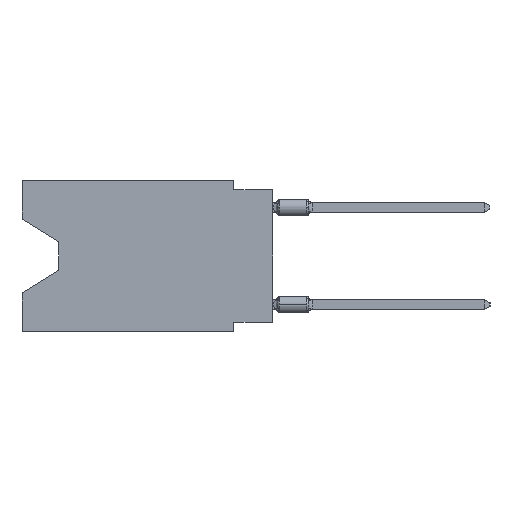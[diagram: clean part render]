
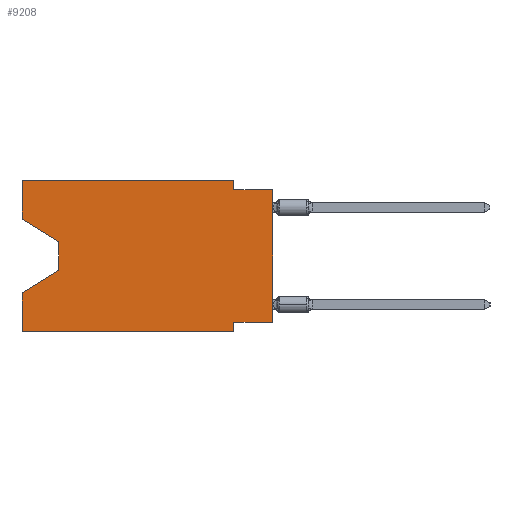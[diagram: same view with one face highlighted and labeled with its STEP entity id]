
A CAD part, left-side view. The second image highlights one B-rep face of the part: STEP entity #9208.
In plain terms, the highlighted planar face has unit normal (-1, 0, 0).
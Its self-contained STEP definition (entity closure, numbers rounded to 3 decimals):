
#1092 = EDGE_CURVE ( 'NONE', #17839, #7920, #7425, .T. ) ;
#1132 = DIRECTION ( 'NONE',  ( 0., -1., 0. ) ) ;
#1654 = VECTOR ( 'NONE', #2284, 1000. ) ;
#1678 = DIRECTION ( 'NONE',  ( 0., -1., 0. ) ) ;
#2079 = CARTESIAN_POINT ( 'NONE',  ( 0., 2.54, -9.906 ) ) ;
#2284 = DIRECTION ( 'NONE',  ( 0., 0., 1. ) ) ;
#3123 = VECTOR ( 'NONE', #14315, 1000. ) ;
#3197 = FACE_OUTER_BOUND ( 'NONE', #29894, .T. ) ;
#4047 = LINE ( 'NONE', #12898, #30364 ) ;
#4243 = CARTESIAN_POINT ( 'NONE',  ( 0., 13.97, -4.013 ) ) ;
#4331 = LINE ( 'NONE', #28984, #28839 ) ;
#4496 = VECTOR ( 'NONE', #22997, 1000. ) ;
#4608 = VERTEX_POINT ( 'NONE', #38751 ) ;
#5410 = CARTESIAN_POINT ( 'NONE',  ( 0., 0., -9.271 ) ) ;
#5603 = CARTESIAN_POINT ( 'NONE',  ( 0., 2.54, 0. ) ) ;
#5713 = CARTESIAN_POINT ( 'NONE',  ( 0., 13.97, -4.013 ) ) ;
#6587 = VECTOR ( 'NONE', #21639, 1000. ) ;
#7382 = VERTEX_POINT ( 'NONE', #35926 ) ;
#7425 = LINE ( 'NONE', #31873, #18852 ) ;
#7735 = DIRECTION ( 'NONE',  ( 0., 0., 1. ) ) ;
#7851 = VERTEX_POINT ( 'NONE', #23849 ) ;
#7920 = VERTEX_POINT ( 'NONE', #11840 ) ;
#7927 = CARTESIAN_POINT ( 'NONE',  ( 0., 0., 0. ) ) ;
#8075 = ORIENTED_EDGE ( 'NONE', *, *, #13387, .F. ) ;
#8241 = DIRECTION ( 'NONE',  ( 0., 1., 0. ) ) ;
#8777 = VERTEX_POINT ( 'NONE', #5713 ) ;
#9208 = ADVANCED_FACE ( 'NONE', ( #3197 ), #38724, .F. ) ;
#9430 = LINE ( 'NONE', #28062, #6587 ) ;
#10078 = DIRECTION ( 'NONE',  ( 0., -1., 0. ) ) ;
#10311 = EDGE_CURVE ( 'NONE', #7920, #22312, #16920, .T. ) ;
#10319 = CARTESIAN_POINT ( 'NONE',  ( 0., 2.54, -9.271 ) ) ;
#10396 = EDGE_CURVE ( 'NONE', #4608, #18197, #26857, .T. ) ;
#11307 = DIRECTION ( 'NONE',  ( 1., 0., 0. ) ) ;
#11518 = LINE ( 'NONE', #2079, #3123 ) ;
#11639 = ORIENTED_EDGE ( 'NONE', *, *, #39117, .T. ) ;
#11840 = CARTESIAN_POINT ( 'NONE',  ( 0., 16.383, 0. ) ) ;
#11887 = VECTOR ( 'NONE', #22679, 1000. ) ;
#11985 = VERTEX_POINT ( 'NONE', #32824 ) ;
#12012 = CARTESIAN_POINT ( 'NONE',  ( 0., 0., -0.635 ) ) ;
#12062 = CARTESIAN_POINT ( 'NONE',  ( 0., 16.383, -2.546 ) ) ;
#12454 = CARTESIAN_POINT ( 'NONE',  ( 0., 16.383, -2.546 ) ) ;
#12898 = CARTESIAN_POINT ( 'NONE',  ( 0., 16.383, -9.906 ) ) ;
#12964 = ORIENTED_EDGE ( 'NONE', *, *, #27680, .T. ) ;
#12980 = CARTESIAN_POINT ( 'NONE',  ( 0., 16.383, -9.906 ) ) ;
#13083 = LINE ( 'NONE', #4243, #11887 ) ;
#13387 = EDGE_CURVE ( 'NONE', #16856, #38138, #4331, .T. ) ;
#13941 = LINE ( 'NONE', #31961, #1654 ) ;
#14102 = ORIENTED_EDGE ( 'NONE', *, *, #10311, .F. ) ;
#14315 = DIRECTION ( 'NONE',  ( 0., 0., -1. ) ) ;
#14925 = ORIENTED_EDGE ( 'NONE', *, *, #33185, .F. ) ;
#14949 = EDGE_CURVE ( 'NONE', #7851, #11985, #9430, .T. ) ;
#16289 = ORIENTED_EDGE ( 'NONE', *, *, #37319, .T. ) ;
#16373 = ORIENTED_EDGE ( 'NONE', *, *, #30024, .F. ) ;
#16856 = VERTEX_POINT ( 'NONE', #20951 ) ;
#16912 = ORIENTED_EDGE ( 'NONE', *, *, #10396, .F. ) ;
#16920 = LINE ( 'NONE', #29137, #25562 ) ;
#17839 = VERTEX_POINT ( 'NONE', #12062 ) ;
#17998 = VERTEX_POINT ( 'NONE', #12980 ) ;
#18197 = VERTEX_POINT ( 'NONE', #10319 ) ;
#18852 = VECTOR ( 'NONE', #29668, 1000. ) ;
#19209 = ORIENTED_EDGE ( 'NONE', *, *, #38337, .F. ) ;
#20453 = VECTOR ( 'NONE', #8241, 1000. ) ;
#20951 = CARTESIAN_POINT ( 'NONE',  ( 0., 2.54, -0.635 ) ) ;
#21639 = DIRECTION ( 'NONE',  ( 0., 0.855, -0.519 ) ) ;
#22312 = VERTEX_POINT ( 'NONE', #5603 ) ;
#22679 = DIRECTION ( 'NONE',  ( 0., 0., -1. ) ) ;
#22997 = DIRECTION ( 'NONE',  ( 0., 0., -1. ) ) ;
#23153 = LINE ( 'NONE', #7927, #27807 ) ;
#23849 = CARTESIAN_POINT ( 'NONE',  ( 0., 13.97, -5.893 ) ) ;
#25562 = VECTOR ( 'NONE', #1678, 1000. ) ;
#26148 = AXIS2_PLACEMENT_3D ( 'NONE', #38933, #11307, #30662 ) ;
#26438 = EDGE_CURVE ( 'NONE', #4608, #38138, #23153, .T. ) ;
#26857 = LINE ( 'NONE', #5410, #20453 ) ;
#27680 = EDGE_CURVE ( 'NONE', #8777, #7851, #13083, .T. ) ;
#27807 = VECTOR ( 'NONE', #7735, 1000. ) ;
#28062 = CARTESIAN_POINT ( 'NONE',  ( 0., 13.97, -5.893 ) ) ;
#28080 = LINE ( 'NONE', #12454, #35578 ) ;
#28605 = LINE ( 'NONE', #38008, #4496 ) ;
#28839 = VECTOR ( 'NONE', #1132, 1000. ) ;
#28984 = CARTESIAN_POINT ( 'NONE',  ( 0., 0., -0.635 ) ) ;
#29137 = CARTESIAN_POINT ( 'NONE',  ( 0., 16.383, 0. ) ) ;
#29668 = DIRECTION ( 'NONE',  ( 0., 0., 1. ) ) ;
#29894 = EDGE_LOOP ( 'NONE', ( #11639, #12964, #30260, #19209, #16289, #16373, #16912, #32960, #8075, #14925, #14102, #38620 ) ) ;
#30024 = EDGE_CURVE ( 'NONE', #18197, #7382, #11518, .T. ) ;
#30260 = ORIENTED_EDGE ( 'NONE', *, *, #14949, .T. ) ;
#30364 = VECTOR ( 'NONE', #10078, 1000. ) ;
#30662 = DIRECTION ( 'NONE',  ( 0., 0., -1. ) ) ;
#31873 = CARTESIAN_POINT ( 'NONE',  ( 0., 16.383, 0. ) ) ;
#31961 = CARTESIAN_POINT ( 'NONE',  ( 0., 16.383, 0. ) ) ;
#32824 = CARTESIAN_POINT ( 'NONE',  ( 0., 16.383, -7.36 ) ) ;
#32960 = ORIENTED_EDGE ( 'NONE', *, *, #26438, .T. ) ;
#33185 = EDGE_CURVE ( 'NONE', #22312, #16856, #28605, .T. ) ;
#35578 = VECTOR ( 'NONE', #36886, 1000. ) ;
#35926 = CARTESIAN_POINT ( 'NONE',  ( 0., 2.54, -9.906 ) ) ;
#36886 = DIRECTION ( 'NONE',  ( 0., -0.855, -0.519 ) ) ;
#37319 = EDGE_CURVE ( 'NONE', #17998, #7382, #4047, .T. ) ;
#38008 = CARTESIAN_POINT ( 'NONE',  ( 0., 2.54, 0. ) ) ;
#38138 = VERTEX_POINT ( 'NONE', #12012 ) ;
#38337 = EDGE_CURVE ( 'NONE', #17998, #11985, #13941, .T. ) ;
#38620 = ORIENTED_EDGE ( 'NONE', *, *, #1092, .F. ) ;
#38724 = PLANE ( 'NONE',  #26148 ) ;
#38751 = CARTESIAN_POINT ( 'NONE',  ( 0., 0., -9.271 ) ) ;
#38933 = CARTESIAN_POINT ( 'NONE',  ( 0., 16.383, 0. ) ) ;
#39117 = EDGE_CURVE ( 'NONE', #17839, #8777, #28080, .T. ) ;
